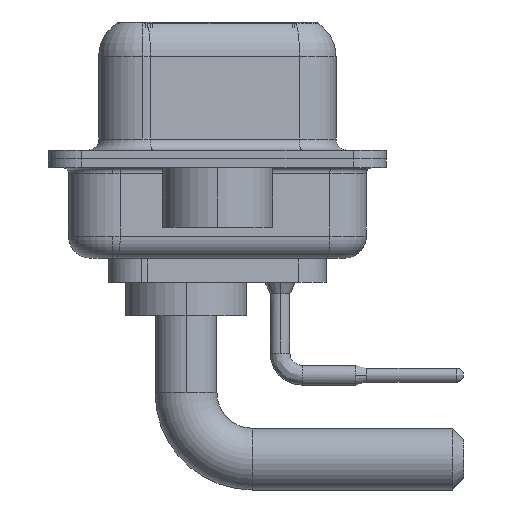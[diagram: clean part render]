
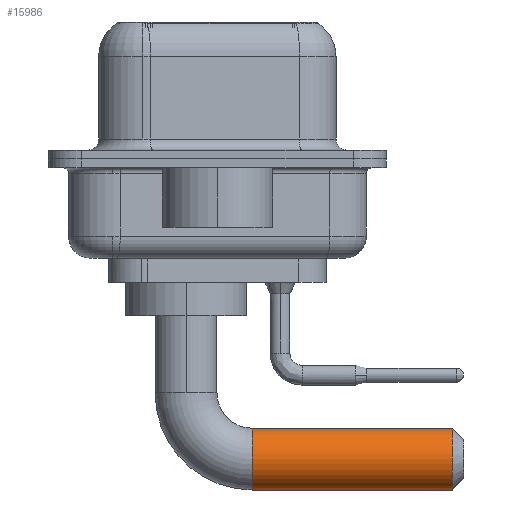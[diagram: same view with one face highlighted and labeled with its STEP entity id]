
A CAD part, left-side view. The second image highlights one B-rep face of the part: STEP entity #15986.
In plain terms, the highlighted cylindrical face has radius 1.4 mm (diameter 2.8 mm), a partial arc.
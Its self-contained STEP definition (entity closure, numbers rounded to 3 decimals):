
#217 = VERTEX_POINT ( 'NONE', #16079 ) ;
#1403 = DIRECTION ( 'NONE',  ( 0., 0., -1. ) ) ;
#1507 = CARTESIAN_POINT ( 'NONE',  ( 0., -12.07, -6.5 ) ) ;
#3649 = CARTESIAN_POINT ( 'NONE',  ( 0., -12.07, -7.9 ) ) ;
#4593 = VECTOR ( 'NONE', #8499, 1000. ) ;
#5155 = LINE ( 'NONE', #11481, #6832 ) ;
#5186 = CARTESIAN_POINT ( 'NONE',  ( 0., -3., -5.1 ) ) ;
#6591 = CARTESIAN_POINT ( 'NONE',  ( 0., -3., -6.5 ) ) ;
#6703 = CARTESIAN_POINT ( 'NONE',  ( 0., -3., -7.9 ) ) ;
#6809 = ORIENTED_EDGE ( 'NONE', *, *, #17048, .T. ) ;
#6832 = VECTOR ( 'NONE', #17977, 1000. ) ;
#6885 = CIRCLE ( 'NONE', #19839, 1.4 ) ;
#6979 = CYLINDRICAL_SURFACE ( 'NONE', #16919, 1.4 ) ;
#7675 = VERTEX_POINT ( 'NONE', #6703 ) ;
#7910 = ORIENTED_EDGE ( 'NONE', *, *, #11055, .T. ) ;
#8499 = DIRECTION ( 'NONE',  ( 0., -1., 0. ) ) ;
#10009 = DIRECTION ( 'NONE',  ( 0., -1., 0. ) ) ;
#10069 = EDGE_CURVE ( 'NONE', #7675, #21041, #5155, .T. ) ;
#10293 = DIRECTION ( 'NONE',  ( 0., -1., 0. ) ) ;
#10545 = CARTESIAN_POINT ( 'NONE',  ( 0., -12.07, -5.1 ) ) ;
#11045 = ORIENTED_EDGE ( 'NONE', *, *, #15389, .F. ) ;
#11055 = EDGE_CURVE ( 'NONE', #217, #7675, #6885, .T. ) ;
#11481 = CARTESIAN_POINT ( 'NONE',  ( 0., -3., -7.9 ) ) ;
#11929 = EDGE_LOOP ( 'NONE', ( #11045, #7910, #18690, #6809 ) ) ;
#13206 = DIRECTION ( 'NONE',  ( 0., 1., 0. ) ) ;
#13320 = LINE ( 'NONE', #5186, #4593 ) ;
#13517 = CARTESIAN_POINT ( 'NONE',  ( 0., -3., -6.5 ) ) ;
#15102 = VERTEX_POINT ( 'NONE', #10545 ) ;
#15125 = FACE_OUTER_BOUND ( 'NONE', #11929, .T. ) ;
#15230 = DIRECTION ( 'NONE',  ( 0., 0., -1. ) ) ;
#15389 = EDGE_CURVE ( 'NONE', #217, #15102, #13320, .T. ) ;
#15986 = ADVANCED_FACE ( 'NONE', ( #15125 ), #6979, .T. ) ;
#16079 = CARTESIAN_POINT ( 'NONE',  ( 0., -3., -5.1 ) ) ;
#16919 = AXIS2_PLACEMENT_3D ( 'NONE', #13517, #10293, #15230 ) ;
#17048 = EDGE_CURVE ( 'NONE', #21041, #15102, #18995, .T. ) ;
#17977 = DIRECTION ( 'NONE',  ( 0., -1., 0. ) ) ;
#18005 = DIRECTION ( 'NONE',  ( -1., 0., 0. ) ) ;
#18690 = ORIENTED_EDGE ( 'NONE', *, *, #10069, .T. ) ;
#18995 = CIRCLE ( 'NONE', #20011, 1.4 ) ;
#19839 = AXIS2_PLACEMENT_3D ( 'NONE', #6591, #10009, #18005 ) ;
#20011 = AXIS2_PLACEMENT_3D ( 'NONE', #1507, #13206, #1403 ) ;
#21041 = VERTEX_POINT ( 'NONE', #3649 ) ;
